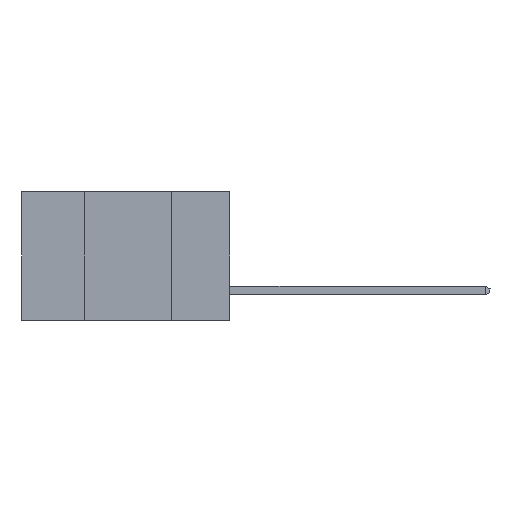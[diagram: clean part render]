
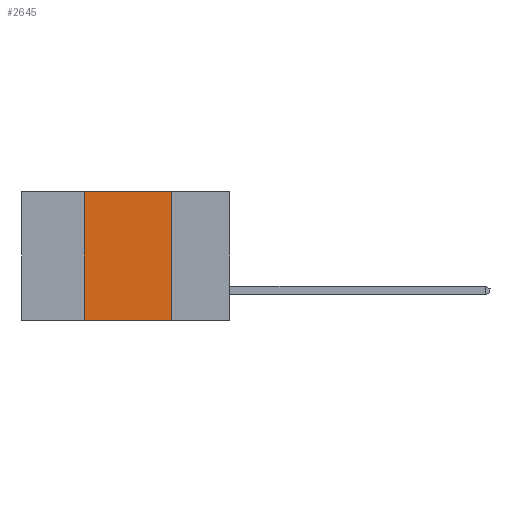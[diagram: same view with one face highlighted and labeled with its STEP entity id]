
A CAD part, left-side view. The second image highlights one B-rep face of the part: STEP entity #2645.
In plain terms, the highlighted planar face has unit normal (-1, 0, 0).
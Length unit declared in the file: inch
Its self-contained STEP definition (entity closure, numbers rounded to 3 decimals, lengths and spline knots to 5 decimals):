
#204 = VECTOR ( 'NONE', #12643, 39.37008 ) ;
#580 = CARTESIAN_POINT ( 'NONE',  ( 0., 0.42, -0.37 ) ) ;
#1250 = VERTEX_POINT ( 'NONE', #1975 ) ;
#1357 = DIRECTION ( 'NONE',  ( 0., 0., -1. ) ) ;
#1793 = DIRECTION ( 'NONE',  ( 0., 0., 1. ) ) ;
#1929 = ORIENTED_EDGE ( 'NONE', *, *, #11525, .F. ) ;
#1975 = CARTESIAN_POINT ( 'NONE',  ( 0., 0.42, -0.37 ) ) ;
#2079 = DIRECTION ( 'NONE',  ( 1., 0., 0. ) ) ;
#2131 = EDGE_LOOP ( 'NONE', ( #1929, #8429, #3996, #8091 ) ) ;
#2645 = ADVANCED_FACE ( 'NONE', ( #3657 ), #9129, .F. ) ;
#3657 = FACE_OUTER_BOUND ( 'NONE', #2131, .T. ) ;
#3996 = ORIENTED_EDGE ( 'NONE', *, *, #5986, .F. ) ;
#4462 = EDGE_CURVE ( 'NONE', #7361, #9305, #11984, .T. ) ;
#4689 = VECTOR ( 'NONE', #1357, 39.37008 ) ;
#5204 = LINE ( 'NONE', #9106, #4689 ) ;
#5986 = EDGE_CURVE ( 'NONE', #1250, #7361, #7122, .T. ) ;
#6602 = DIRECTION ( 'NONE',  ( 0., -1., 0. ) ) ;
#7122 = LINE ( 'NONE', #580, #16785 ) ;
#7361 = VERTEX_POINT ( 'NONE', #8697 ) ;
#7739 = CARTESIAN_POINT ( 'NONE',  ( 0., 0.6, 0. ) ) ;
#7894 = CARTESIAN_POINT ( 'NONE',  ( 0., 0.6, 0. ) ) ;
#8091 = ORIENTED_EDGE ( 'NONE', *, *, #10318, .T. ) ;
#8429 = ORIENTED_EDGE ( 'NONE', *, *, #4462, .F. ) ;
#8697 = CARTESIAN_POINT ( 'NONE',  ( 0., 0.42, 0. ) ) ;
#9106 = CARTESIAN_POINT ( 'NONE',  ( 0., 0.17, -0.37 ) ) ;
#9129 = PLANE ( 'NONE',  #13645 ) ;
#9305 = VERTEX_POINT ( 'NONE', #11935 ) ;
#9436 = CARTESIAN_POINT ( 'NONE',  ( 0., 0.17, -0.37 ) ) ;
#10318 = EDGE_CURVE ( 'NONE', #1250, #16347, #15240, .T. ) ;
#10542 = VECTOR ( 'NONE', #6602, 39.37008 ) ;
#11525 = EDGE_CURVE ( 'NONE', #9305, #16347, #5204, .T. ) ;
#11935 = CARTESIAN_POINT ( 'NONE',  ( 0., 0.17, 0. ) ) ;
#11984 = LINE ( 'NONE', #7894, #10542 ) ;
#12643 = DIRECTION ( 'NONE',  ( 0., -1., 0. ) ) ;
#13645 = AXIS2_PLACEMENT_3D ( 'NONE', #7739, #2079, #15549 ) ;
#15240 = LINE ( 'NONE', #16628, #204 ) ;
#15549 = DIRECTION ( 'NONE',  ( 0., 0., -1. ) ) ;
#16347 = VERTEX_POINT ( 'NONE', #9436 ) ;
#16628 = CARTESIAN_POINT ( 'NONE',  ( 0., 0.6, -0.37 ) ) ;
#16785 = VECTOR ( 'NONE', #1793, 39.37008 ) ;
